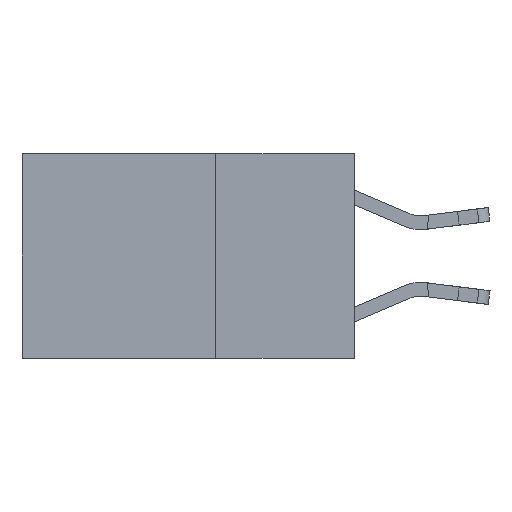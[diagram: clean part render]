
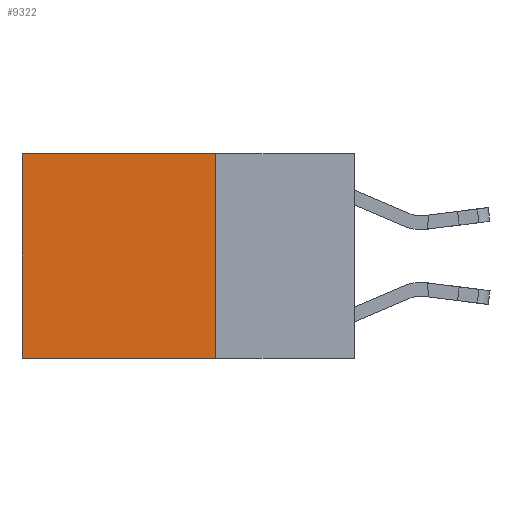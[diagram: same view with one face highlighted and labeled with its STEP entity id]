
A CAD part, left-side view. The second image highlights one B-rep face of the part: STEP entity #9322.
In plain terms, the highlighted planar face has unit normal (-1, 0, 0).
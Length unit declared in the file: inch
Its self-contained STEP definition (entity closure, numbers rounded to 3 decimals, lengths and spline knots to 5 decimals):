
#658 = DIRECTION ( 'NONE',  ( 0., 1., 0. ) ) ;
#1165 = VERTEX_POINT ( 'NONE', #8152 ) ;
#2168 = LINE ( 'NONE', #10358, #9346 ) ;
#2263 = PLANE ( 'NONE',  #6368 ) ;
#2289 = EDGE_LOOP ( 'NONE', ( #4360, #3181, #4939, #4992 ) ) ;
#2802 = FACE_OUTER_BOUND ( 'NONE', #2289, .T. ) ;
#3181 = ORIENTED_EDGE ( 'NONE', *, *, #10252, .F. ) ;
#3323 = DIRECTION ( 'NONE',  ( 0., 0., -1. ) ) ;
#3791 = CARTESIAN_POINT ( 'NONE',  ( 0.2625, 0.6, 0. ) ) ;
#4085 = VERTEX_POINT ( 'NONE', #10147 ) ;
#4123 = CARTESIAN_POINT ( 'NONE',  ( 0.2625, 0.25, 0. ) ) ;
#4348 = CARTESIAN_POINT ( 'NONE',  ( 0.2625, 0.25, 0. ) ) ;
#4360 = ORIENTED_EDGE ( 'NONE', *, *, #8096, .T. ) ;
#4520 = VECTOR ( 'NONE', #9024, 39.37008 ) ;
#4548 = VERTEX_POINT ( 'NONE', #9088 ) ;
#4814 = DIRECTION ( 'NONE',  ( 0., 0., -1. ) ) ;
#4939 = ORIENTED_EDGE ( 'NONE', *, *, #6994, .F. ) ;
#4992 = ORIENTED_EDGE ( 'NONE', *, *, #11100, .T. ) ;
#5116 = DIRECTION ( 'NONE',  ( 0., 0., -1. ) ) ;
#6259 = LINE ( 'NONE', #9908, #11069 ) ;
#6368 = AXIS2_PLACEMENT_3D ( 'NONE', #4123, #10627, #5116 ) ;
#6884 = VECTOR ( 'NONE', #658, 39.37008 ) ;
#6994 = EDGE_CURVE ( 'NONE', #1165, #4548, #2168, .T. ) ;
#7458 = VERTEX_POINT ( 'NONE', #3791 ) ;
#8096 = EDGE_CURVE ( 'NONE', #7458, #4085, #6259, .T. ) ;
#8152 = CARTESIAN_POINT ( 'NONE',  ( 0.2625, 0.25, 0. ) ) ;
#9024 = DIRECTION ( 'NONE',  ( 0., 1., 0. ) ) ;
#9088 = CARTESIAN_POINT ( 'NONE',  ( 0.2625, 0.25, -0.37 ) ) ;
#9322 = ADVANCED_FACE ( 'NONE', ( #2802 ), #2263, .F. ) ;
#9346 = VECTOR ( 'NONE', #4814, 39.37008 ) ;
#9383 = LINE ( 'NONE', #11670, #6884 ) ;
#9509 = LINE ( 'NONE', #4348, #4520 ) ;
#9908 = CARTESIAN_POINT ( 'NONE',  ( 0.2625, 0.6, 0. ) ) ;
#10147 = CARTESIAN_POINT ( 'NONE',  ( 0.2625, 0.6, -0.37 ) ) ;
#10252 = EDGE_CURVE ( 'NONE', #4548, #4085, #9383, .T. ) ;
#10358 = CARTESIAN_POINT ( 'NONE',  ( 0.2625, 0.25, 0. ) ) ;
#10627 = DIRECTION ( 'NONE',  ( 1., 0., 0. ) ) ;
#11069 = VECTOR ( 'NONE', #3323, 39.37008 ) ;
#11100 = EDGE_CURVE ( 'NONE', #1165, #7458, #9509, .T. ) ;
#11670 = CARTESIAN_POINT ( 'NONE',  ( 0.2625, 0.25, -0.37 ) ) ;
